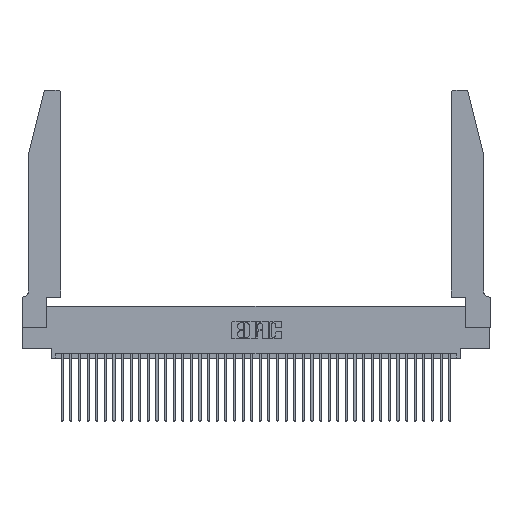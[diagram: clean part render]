
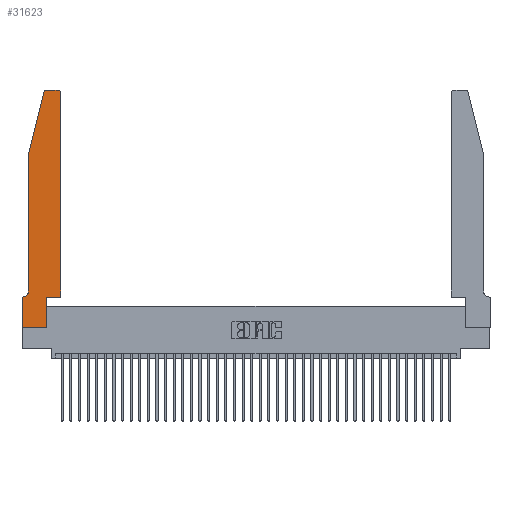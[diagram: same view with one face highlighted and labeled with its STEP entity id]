
A CAD part, top view. The second image highlights one B-rep face of the part: STEP entity #31623.
In plain terms, the highlighted planar face has unit normal (0, 0, 1).
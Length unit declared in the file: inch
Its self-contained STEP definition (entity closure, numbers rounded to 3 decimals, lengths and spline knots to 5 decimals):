
#1053 = EDGE_CURVE ( 'NONE', #32996, #37131, #29042, .T. ) ;
#1544 = DIRECTION ( 'NONE',  ( -1., 0., 0. ) ) ;
#1600 = LINE ( 'NONE', #15859, #33900 ) ;
#2331 = LINE ( 'NONE', #31196, #10722 ) ;
#2953 = CARTESIAN_POINT ( 'NONE',  ( 0.4205, 2.72, 0.37 ) ) ;
#3162 = ORIENTED_EDGE ( 'NONE', *, *, #20535, .T. ) ;
#3317 = DIRECTION ( 'NONE',  ( 1., 0., 0. ) ) ;
#3333 = AXIS2_PLACEMENT_3D ( 'NONE', #38922, #20413, #1544 ) ;
#3563 = EDGE_CURVE ( 'NONE', #27315, #39438, #31548, .T. ) ;
#3895 = EDGE_CURVE ( 'NONE', #38001, #27315, #28129, .T. ) ;
#3993 = CARTESIAN_POINT ( 'NONE',  ( 0.0755, 2., 0.37 ) ) ;
#4175 = ORIENTED_EDGE ( 'NONE', *, *, #39343, .T. ) ;
#4558 = LINE ( 'NONE', #32106, #8488 ) ;
#4770 = CARTESIAN_POINT ( 'NONE',  ( 0., 0.35, 0.37 ) ) ;
#4807 = VERTEX_POINT ( 'NONE', #9549 ) ;
#6018 = VECTOR ( 'NONE', #31872, 39.37008 ) ;
#6144 = DIRECTION ( 'NONE',  ( 1., 0., 0. ) ) ;
#7677 = PLANE ( 'NONE',  #39351 ) ;
#7802 = EDGE_CURVE ( 'NONE', #39438, #10197, #39155, .T. ) ;
#7807 = DIRECTION ( 'NONE',  ( 1., 0., 0. ) ) ;
#7876 = LINE ( 'NONE', #16068, #23588 ) ;
#8290 = CARTESIAN_POINT ( 'NONE',  ( 0.0755, 2., 0.37 ) ) ;
#8488 = VECTOR ( 'NONE', #13433, 39.37008 ) ;
#8902 = FACE_OUTER_BOUND ( 'NONE', #22344, .T. ) ;
#9549 = CARTESIAN_POINT ( 'NONE',  ( 0.25487, 2.72718, 0.37 ) ) ;
#9625 = CARTESIAN_POINT ( 'NONE',  ( 0.4505, 0.35, 0.37 ) ) ;
#10197 = VERTEX_POINT ( 'NONE', #29480 ) ;
#10426 = EDGE_CURVE ( 'NONE', #28915, #32996, #2331, .T. ) ;
#10722 = VECTOR ( 'NONE', #18582, 39.37008 ) ;
#11438 = ORIENTED_EDGE ( 'NONE', *, *, #38363, .T. ) ;
#11758 = ORIENTED_EDGE ( 'NONE', *, *, #37113, .T. ) ;
#12695 = CIRCLE ( 'NONE', #3333, 0.07 ) ;
#12736 = ORIENTED_EDGE ( 'NONE', *, *, #30704, .T. ) ;
#12918 = DIRECTION ( 'NONE',  ( -0.239, -0.971, 0. ) ) ;
#13433 = DIRECTION ( 'NONE',  ( -1., 0., 0. ) ) ;
#15710 = VECTOR ( 'NONE', #19704, 39.37008 ) ;
#15859 = CARTESIAN_POINT ( 'NONE',  ( 0., 0., 0.37 ) ) ;
#16049 = ORIENTED_EDGE ( 'NONE', *, *, #1053, .T. ) ;
#16068 = CARTESIAN_POINT ( 'NONE',  ( 0.0755, 2., 0.37 ) ) ;
#17468 = CARTESIAN_POINT ( 'NONE',  ( 0.2865, 0.35, 0.37 ) ) ;
#18053 = CARTESIAN_POINT ( 'NONE',  ( 0.0055, 0.35, 0.37 ) ) ;
#18174 = CARTESIAN_POINT ( 'NONE',  ( 0.2865, 0., 0.37 ) ) ;
#18310 = ORIENTED_EDGE ( 'NONE', *, *, #10426, .T. ) ;
#18396 = DIRECTION ( 'NONE',  ( 0., 0., 1. ) ) ;
#18582 = DIRECTION ( 'NONE',  ( -1., 0., 0. ) ) ;
#19534 = CARTESIAN_POINT ( 'NONE',  ( 0.4505, 0.35, 0.37 ) ) ;
#19704 = DIRECTION ( 'NONE',  ( 0., -1., 0. ) ) ;
#19737 = CIRCLE ( 'NONE', #21870, 0.03 ) ;
#20413 = DIRECTION ( 'NONE',  ( 0., 0., -1. ) ) ;
#20535 = EDGE_CURVE ( 'NONE', #4807, #30433, #7876, .T. ) ;
#20924 = VERTEX_POINT ( 'NONE', #28286 ) ;
#21870 = AXIS2_PLACEMENT_3D ( 'NONE', #36929, #18396, #40042 ) ;
#22344 = EDGE_LOOP ( 'NONE', ( #11758, #11438, #3162, #4175, #33886, #18310, #16049, #12736, #28794, #39928, #37344, #27209 ) ) ;
#22751 = CARTESIAN_POINT ( 'NONE',  ( 0., 0., 0.37 ) ) ;
#22948 = CARTESIAN_POINT ( 'NONE',  ( 0.0755, 0.42, 0.37 ) ) ;
#23588 = VECTOR ( 'NONE', #12918, 39.37008 ) ;
#24058 = DIRECTION ( 'NONE',  ( 0., -1., 0. ) ) ;
#24944 = DIRECTION ( 'NONE',  ( 0., 0., 1. ) ) ;
#25276 = DIRECTION ( 'NONE',  ( 1., 0., 0. ) ) ;
#26106 = CARTESIAN_POINT ( 'NONE',  ( 0.4505, 0.35, 0.37 ) ) ;
#26600 = DIRECTION ( 'NONE',  ( 0., 0., 1. ) ) ;
#26625 = EDGE_CURVE ( 'NONE', #10197, #29586, #37154, .T. ) ;
#27209 = ORIENTED_EDGE ( 'NONE', *, *, #26625, .T. ) ;
#27315 = VERTEX_POINT ( 'NONE', #37937 ) ;
#28129 = LINE ( 'NONE', #17468, #36317 ) ;
#28286 = CARTESIAN_POINT ( 'NONE',  ( 0.284, 2.75, 0.37 ) ) ;
#28794 = ORIENTED_EDGE ( 'NONE', *, *, #3895, .T. ) ;
#28915 = VERTEX_POINT ( 'NONE', #18053 ) ;
#29042 = LINE ( 'NONE', #33390, #36245 ) ;
#29480 = CARTESIAN_POINT ( 'NONE',  ( 0.4505, 2.72, 0.37 ) ) ;
#29586 = VERTEX_POINT ( 'NONE', #30654 ) ;
#30433 = VERTEX_POINT ( 'NONE', #8290 ) ;
#30654 = CARTESIAN_POINT ( 'NONE',  ( 0.4205, 2.75, 0.37 ) ) ;
#30704 = EDGE_CURVE ( 'NONE', #37131, #38001, #1600, .T. ) ;
#31196 = CARTESIAN_POINT ( 'NONE',  ( 0.0755, 0.35, 0.37 ) ) ;
#31548 = LINE ( 'NONE', #9625, #39726 ) ;
#31623 = ADVANCED_FACE ( 'NONE', ( #8902 ), #7677, .T. ) ;
#31872 = DIRECTION ( 'NONE',  ( 0., 1., 0. ) ) ;
#32106 = CARTESIAN_POINT ( 'NONE',  ( 0.2605, 2.75, 0.37 ) ) ;
#32996 = VERTEX_POINT ( 'NONE', #4770 ) ;
#33390 = CARTESIAN_POINT ( 'NONE',  ( 0., 0., 0.37 ) ) ;
#33531 = EDGE_CURVE ( 'NONE', #39368, #28915, #12695, .T. ) ;
#33886 = ORIENTED_EDGE ( 'NONE', *, *, #33531, .T. ) ;
#33900 = VECTOR ( 'NONE', #3317, 39.37008 ) ;
#35742 = CARTESIAN_POINT ( 'NONE',  ( 0., 0.35, 0.37 ) ) ;
#36245 = VECTOR ( 'NONE', #24058, 39.37008 ) ;
#36317 = VECTOR ( 'NONE', #39135, 39.37008 ) ;
#36929 = CARTESIAN_POINT ( 'NONE',  ( 0.284, 2.72, 0.37 ) ) ;
#37113 = EDGE_CURVE ( 'NONE', #29586, #20924, #4558, .T. ) ;
#37131 = VERTEX_POINT ( 'NONE', #22751 ) ;
#37154 = CIRCLE ( 'NONE', #37924, 0.03 ) ;
#37344 = ORIENTED_EDGE ( 'NONE', *, *, #7802, .T. ) ;
#37924 = AXIS2_PLACEMENT_3D ( 'NONE', #2953, #24944, #6144 ) ;
#37937 = CARTESIAN_POINT ( 'NONE',  ( 0.2865, 0.35, 0.37 ) ) ;
#38001 = VERTEX_POINT ( 'NONE', #18174 ) ;
#38363 = EDGE_CURVE ( 'NONE', #20924, #4807, #19737, .T. ) ;
#38922 = CARTESIAN_POINT ( 'NONE',  ( 0.0055, 0.42, 0.37 ) ) ;
#39135 = DIRECTION ( 'NONE',  ( 0., 1., 0. ) ) ;
#39155 = LINE ( 'NONE', #19534, #6018 ) ;
#39343 = EDGE_CURVE ( 'NONE', #30433, #39368, #40453, .T. ) ;
#39351 = AXIS2_PLACEMENT_3D ( 'NONE', #35742, #26600, #7807 ) ;
#39368 = VERTEX_POINT ( 'NONE', #22948 ) ;
#39438 = VERTEX_POINT ( 'NONE', #26106 ) ;
#39726 = VECTOR ( 'NONE', #25276, 39.37008 ) ;
#39928 = ORIENTED_EDGE ( 'NONE', *, *, #3563, .T. ) ;
#40042 = DIRECTION ( 'NONE',  ( 1., 0., 0. ) ) ;
#40453 = LINE ( 'NONE', #3993, #15710 ) ;
